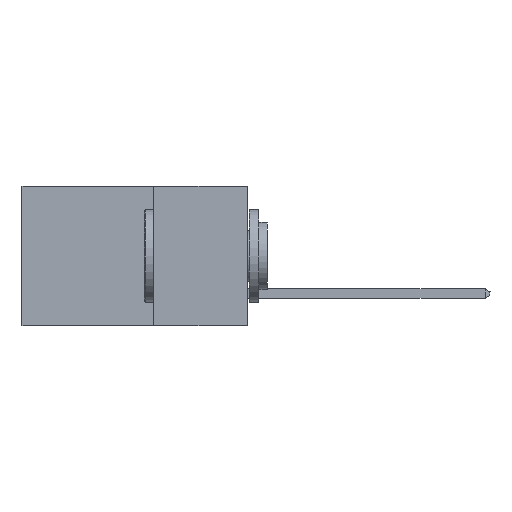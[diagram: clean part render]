
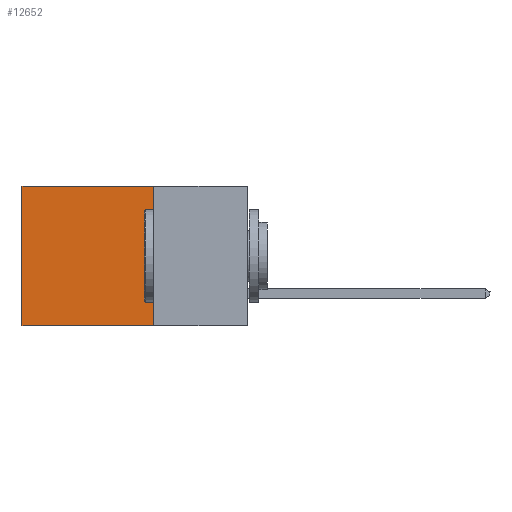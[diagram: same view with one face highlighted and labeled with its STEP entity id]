
A CAD part, left-side view. The second image highlights one B-rep face of the part: STEP entity #12652.
In plain terms, the highlighted planar face has unit normal (-1, 0, 0).
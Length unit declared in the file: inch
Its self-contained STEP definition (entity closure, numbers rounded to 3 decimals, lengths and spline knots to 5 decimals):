
#296 = VECTOR ( 'NONE', #9589, 39.37008 ) ;
#392 = DIRECTION ( 'NONE',  ( 0., 1., 0. ) ) ;
#1418 = CARTESIAN_POINT ( 'NONE',  ( 0.2615, 0.6, -0.37 ) ) ;
#1607 = FACE_OUTER_BOUND ( 'NONE', #8045, .T. ) ;
#1652 = CARTESIAN_POINT ( 'NONE',  ( 0.2615, 0.6, -0.37 ) ) ;
#3549 = LINE ( 'NONE', #15157, #296 ) ;
#5586 = DIRECTION ( 'NONE',  ( 0., 0., -1. ) ) ;
#6168 = ORIENTED_EDGE ( 'NONE', *, *, #6571, .T. ) ;
#6571 = EDGE_CURVE ( 'NONE', #22229, #8780, #3549, .T. ) ;
#7556 = PLANE ( 'NONE',  #23101 ) ;
#7804 = EDGE_CURVE ( 'NONE', #22229, #9194, #14436, .T. ) ;
#7942 = CARTESIAN_POINT ( 'NONE',  ( 0.2615, 0.25, -0.37 ) ) ;
#8045 = EDGE_LOOP ( 'NONE', ( #21437, #22814, #20765, #6168 ) ) ;
#8365 = EDGE_CURVE ( 'NONE', #8780, #14305, #20702, .T. ) ;
#8780 = VERTEX_POINT ( 'NONE', #9065 ) ;
#8997 = DIRECTION ( 'NONE',  ( 0., 0., -1. ) ) ;
#9065 = CARTESIAN_POINT ( 'NONE',  ( 0.2615, 0.6, 0. ) ) ;
#9194 = VERTEX_POINT ( 'NONE', #11477 ) ;
#9589 = DIRECTION ( 'NONE',  ( 0., 1., 0. ) ) ;
#10020 = CARTESIAN_POINT ( 'NONE',  ( 0.2615, 0.25, 0. ) ) ;
#11477 = CARTESIAN_POINT ( 'NONE',  ( 0.2615, 0.25, -0.37 ) ) ;
#11994 = VECTOR ( 'NONE', #392, 39.37008 ) ;
#12652 = ADVANCED_FACE ( 'NONE', ( #1607 ), #7556, .F. ) ;
#13532 = EDGE_CURVE ( 'NONE', #9194, #14305, #17338, .T. ) ;
#13993 = VECTOR ( 'NONE', #16874, 39.37008 ) ;
#14305 = VERTEX_POINT ( 'NONE', #1418 ) ;
#14436 = LINE ( 'NONE', #21968, #14495 ) ;
#14495 = VECTOR ( 'NONE', #8997, 39.37008 ) ;
#15157 = CARTESIAN_POINT ( 'NONE',  ( 0.2615, 0.25, 0. ) ) ;
#16874 = DIRECTION ( 'NONE',  ( 0., 0., -1. ) ) ;
#17338 = LINE ( 'NONE', #7942, #11994 ) ;
#20702 = LINE ( 'NONE', #1652, #13993 ) ;
#20765 = ORIENTED_EDGE ( 'NONE', *, *, #7804, .F. ) ;
#21437 = ORIENTED_EDGE ( 'NONE', *, *, #8365, .T. ) ;
#21968 = CARTESIAN_POINT ( 'NONE',  ( 0.2615, 0.25, -0.37 ) ) ;
#22229 = VERTEX_POINT ( 'NONE', #10020 ) ;
#22246 = DIRECTION ( 'NONE',  ( 1., 0., 0. ) ) ;
#22814 = ORIENTED_EDGE ( 'NONE', *, *, #13532, .F. ) ;
#23101 = AXIS2_PLACEMENT_3D ( 'NONE', #23992, #22246, #5586 ) ;
#23992 = CARTESIAN_POINT ( 'NONE',  ( 0.2615, 0.25, -0.37 ) ) ;
